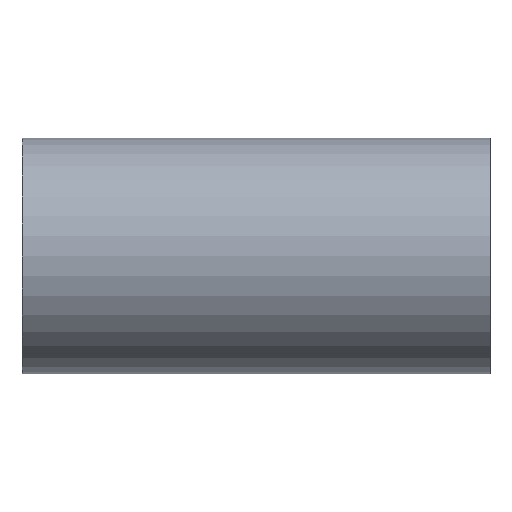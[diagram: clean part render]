
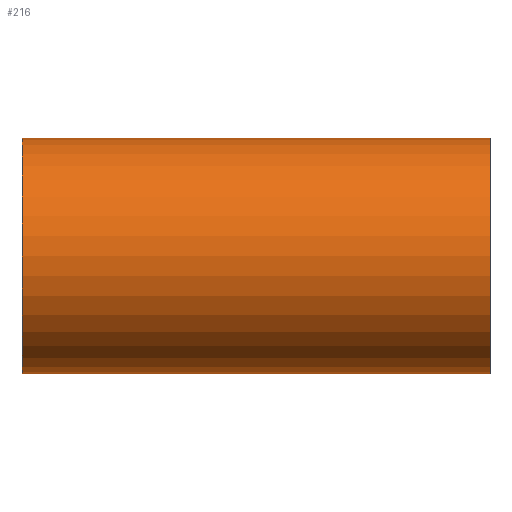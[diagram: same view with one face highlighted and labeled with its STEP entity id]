
A CAD part, front view. The second image highlights one B-rep face of the part: STEP entity #216.
In plain terms, the highlighted cylindrical face has radius 3 mm (diameter 6 mm), a full revolution.
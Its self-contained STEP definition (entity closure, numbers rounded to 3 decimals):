
#73=CARTESIAN_POINT('',(-1.0,0.0,3.0));
#74=VERTEX_POINT('',#73);
#75=CARTESIAN_POINT('',(-1.0,0.0,-3.0));
#76=VERTEX_POINT('',#75);
#77=CARTESIAN_POINT('',(-1.0,0.0,0.0));
#78=DIRECTION('',(-1.0,0.0,0.0));
#79=DIRECTION('',(0.0,-1.0,0.0));
#80=AXIS2_PLACEMENT_3D('',#77,#78,#79);
#81=CIRCLE('',#80,3.0);
#82=EDGE_CURVE('',#74,#76,#81,.T.);
#123=CARTESIAN_POINT('',(0.0,0.0,-3.0));
#124=VERTEX_POINT('',#123);
#131=CARTESIAN_POINT('',(0.0,0.,-3.0));
#132=DIRECTION('',(-1.0,0.0,0.0));
#133=VECTOR('',#132,1.0);
#134=LINE('',#131,#133);
#135=EDGE_CURVE('',#124,#76,#134,.T.);
#170=CARTESIAN_POINT('',(0.0,0.0,3.0));
#171=VERTEX_POINT('',#170);
#172=CARTESIAN_POINT('',(0.0,0.0,3.0));
#173=DIRECTION('',(-1.0,0.0,0.0));
#174=VECTOR('',#173,1.0);
#175=LINE('',#172,#174);
#176=EDGE_CURVE('',#171,#74,#175,.T.);
#188=CARTESIAN_POINT('',(0.0,0.0,0.0));
#189=DIRECTION('',(-1.0,0.0,0.0));
#190=DIRECTION('',(0.0,-1.0,0.0));
#191=AXIS2_PLACEMENT_3D('',#188,#189,#190);
#192=CYLINDRICAL_SURFACE('',#191,3.0);
#193=ORIENTED_EDGE('',*,*,#82,.T.);
#194=ORIENTED_EDGE('',*,*,#135,.F.);
#195=CARTESIAN_POINT('',(0.0,0.0,0.0));
#196=DIRECTION('',(-1.0,0.0,0.0));
#197=DIRECTION('',(0.0,-1.0,0.0));
#198=AXIS2_PLACEMENT_3D('',#195,#196,#197);
#199=CIRCLE('',#198,3.0);
#200=EDGE_CURVE('',#124,#171,#199,.T.);
#201=ORIENTED_EDGE('',*,*,#200,.T.);
#202=ORIENTED_EDGE('',*,*,#176,.T.);
#203=EDGE_LOOP('',(#193,#194,#201,#202));
#204=FACE_OUTER_BOUND('',#203,.T.);
#205=CARTESIAN_POINT('',(-11.9,3.0,0.));
#206=VERTEX_POINT('',#205);
#207=CARTESIAN_POINT('',(-11.9,0.0,0.0));
#208=DIRECTION('',(1.0,0.0,0.0));
#209=DIRECTION('',(0.0,-1.0,0.0));
#210=AXIS2_PLACEMENT_3D('',#207,#208,#209);
#211=CIRCLE('',#210,3.0);
#212=EDGE_CURVE('',#206,#206,#211,.T.);
#213=ORIENTED_EDGE('',*,*,#212,.T.);
#214=EDGE_LOOP('',(#213));
#215=FACE_BOUND('',#214,.T.);
#216=ADVANCED_FACE('',(#204,#215),#192,.T.);
